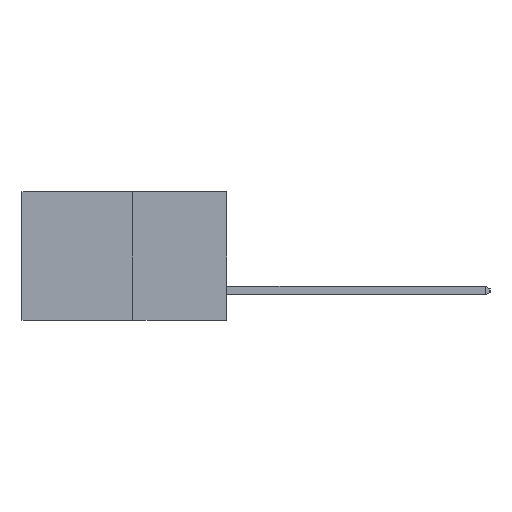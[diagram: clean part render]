
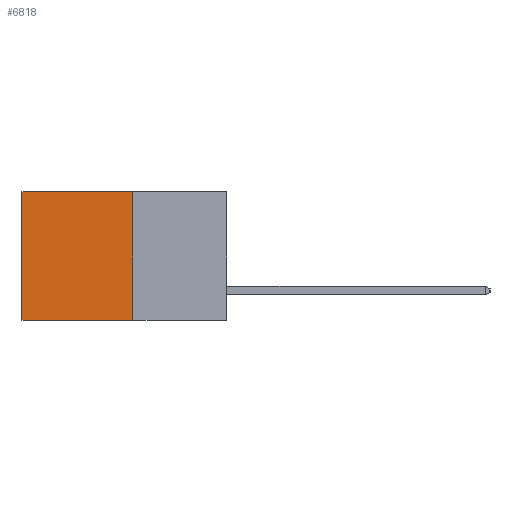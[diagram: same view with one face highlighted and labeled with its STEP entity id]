
A CAD part, left-side view. The second image highlights one B-rep face of the part: STEP entity #6818.
In plain terms, the highlighted planar face has unit normal (-1, 0, 0).
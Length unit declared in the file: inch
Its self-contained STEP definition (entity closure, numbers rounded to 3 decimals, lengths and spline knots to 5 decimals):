
#176 = CARTESIAN_POINT ( 'NONE',  ( 0.277, 0.59, -0.37 ) ) ;
#361 = LINE ( 'NONE', #6667, #7950 ) ;
#387 = LINE ( 'NONE', #3586, #6264 ) ;
#494 = DIRECTION ( 'NONE',  ( 1., 0., 0. ) ) ;
#579 = DIRECTION ( 'NONE',  ( 0., 0., -1. ) ) ;
#855 = EDGE_LOOP ( 'NONE', ( #8241, #3054, #5521, #1299 ) ) ;
#939 = VERTEX_POINT ( 'NONE', #7313 ) ;
#1014 = DIRECTION ( 'NONE',  ( 0., 1., 0. ) ) ;
#1299 = ORIENTED_EDGE ( 'NONE', *, *, #7660, .T. ) ;
#1352 = DIRECTION ( 'NONE',  ( 0., 1., 0. ) ) ;
#2085 = CARTESIAN_POINT ( 'NONE',  ( 0.277, 0.27, -0.37 ) ) ;
#2758 = FACE_OUTER_BOUND ( 'NONE', #855, .T. ) ;
#2839 = DIRECTION ( 'NONE',  ( 0., 0., -1. ) ) ;
#3054 = ORIENTED_EDGE ( 'NONE', *, *, #4897, .F. ) ;
#3163 = CARTESIAN_POINT ( 'NONE',  ( 0.277, 0.27, -0.37 ) ) ;
#3212 = VECTOR ( 'NONE', #1014, 39.37008 ) ;
#3330 = VERTEX_POINT ( 'NONE', #176 ) ;
#3586 = CARTESIAN_POINT ( 'NONE',  ( 0.277, 0.27, -0.37 ) ) ;
#4741 = VERTEX_POINT ( 'NONE', #7959 ) ;
#4799 = CARTESIAN_POINT ( 'NONE',  ( 0.277, 0.27, 0. ) ) ;
#4897 = EDGE_CURVE ( 'NONE', #9678, #3330, #387, .T. ) ;
#5105 = CARTESIAN_POINT ( 'NONE',  ( 0.277, 0.27, -0.37 ) ) ;
#5521 = ORIENTED_EDGE ( 'NONE', *, *, #9374, .F. ) ;
#5881 = DIRECTION ( 'NONE',  ( 0., 0., -1. ) ) ;
#6246 = EDGE_CURVE ( 'NONE', #939, #3330, #361, .T. ) ;
#6264 = VECTOR ( 'NONE', #1352, 39.37008 ) ;
#6553 = AXIS2_PLACEMENT_3D ( 'NONE', #5105, #494, #5881 ) ;
#6667 = CARTESIAN_POINT ( 'NONE',  ( 0.277, 0.59, -0.37 ) ) ;
#6818 = ADVANCED_FACE ( 'NONE', ( #2758 ), #9493, .F. ) ;
#7245 = LINE ( 'NONE', #4799, #3212 ) ;
#7313 = CARTESIAN_POINT ( 'NONE',  ( 0.277, 0.59, 0. ) ) ;
#7429 = LINE ( 'NONE', #2085, #9348 ) ;
#7660 = EDGE_CURVE ( 'NONE', #4741, #939, #7245, .T. ) ;
#7950 = VECTOR ( 'NONE', #579, 39.37008 ) ;
#7959 = CARTESIAN_POINT ( 'NONE',  ( 0.277, 0.27, 0. ) ) ;
#8241 = ORIENTED_EDGE ( 'NONE', *, *, #6246, .T. ) ;
#9348 = VECTOR ( 'NONE', #2839, 39.37008 ) ;
#9374 = EDGE_CURVE ( 'NONE', #4741, #9678, #7429, .T. ) ;
#9493 = PLANE ( 'NONE',  #6553 ) ;
#9678 = VERTEX_POINT ( 'NONE', #3163 ) ;
